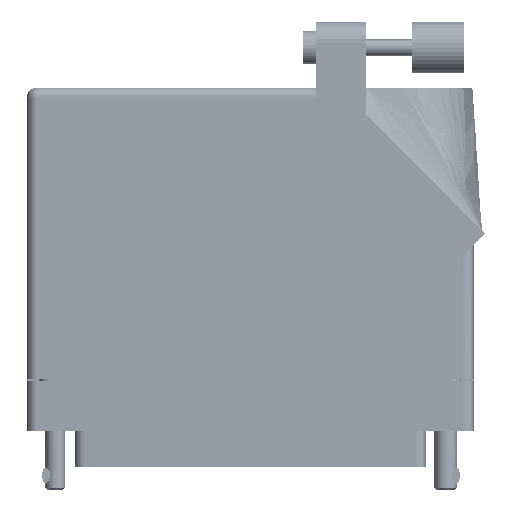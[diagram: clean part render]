
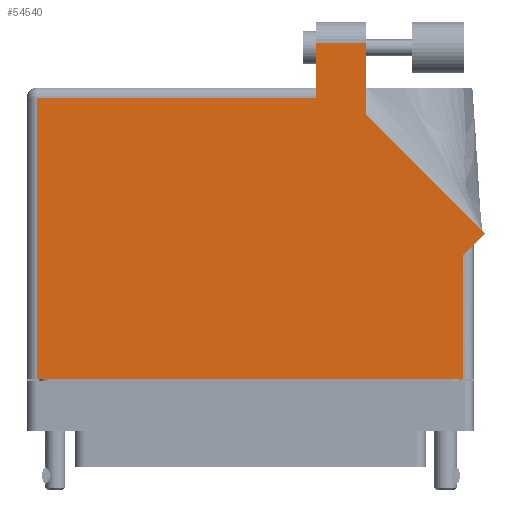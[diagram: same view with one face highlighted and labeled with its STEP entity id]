
A CAD part, front view. The second image highlights one B-rep face of the part: STEP entity #54540.
In plain terms, the highlighted face is planar.
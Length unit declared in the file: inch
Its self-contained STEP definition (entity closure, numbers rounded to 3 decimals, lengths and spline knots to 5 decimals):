
#1193 = CARTESIAN_POINT ( 'NONE',  ( -1.297, -0.1, 0.617 ) ) ;
#1477 = DIRECTION ( 'NONE',  ( -0.707, 0.707, 0. ) ) ;
#1693 = DIRECTION ( 'NONE',  ( -1., 0., 0. ) ) ;
#4612 = CARTESIAN_POINT ( 'NONE',  ( 1.297, 0.653, 0.617 ) ) ;
#4643 = VERTEX_POINT ( 'NONE', #49064 ) ;
#9513 = EDGE_CURVE ( 'NONE', #53875, #79108, #11971, .T. ) ;
#10270 = ORIENTED_EDGE ( 'NONE', *, *, #74179, .T. ) ;
#11971 = LINE ( 'NONE', #51084, #12599 ) ;
#12599 = VECTOR ( 'NONE', #78226, 39.37008 ) ;
#13262 = DIRECTION ( 'NONE',  ( 0., -1., 0. ) ) ;
#16221 = CARTESIAN_POINT ( 'NONE',  ( 0.706, 1.50942, 0.617 ) ) ;
#16449 = CARTESIAN_POINT ( 'NONE',  ( 1.297, -0.1, 0.617 ) ) ;
#17113 = EDGE_CURVE ( 'NONE', #79108, #62182, #32589, .T. ) ;
#20006 = PLANE ( 'NONE',  #80832 ) ;
#21875 = CARTESIAN_POINT ( 'NONE',  ( 1.297, 0.715, 0.617 ) ) ;
#22116 = CARTESIAN_POINT ( 'NONE',  ( -1.359, 1.613, 0.617 ) ) ;
#22216 = VECTOR ( 'NONE', #13262, 39.37008 ) ;
#22302 = EDGE_CURVE ( 'NONE', #73779, #49938, #82548, .T. ) ;
#24360 = DIRECTION ( 'NONE',  ( 0., -1., 0. ) ) ;
#24768 = CARTESIAN_POINT ( 'NONE',  ( 0.399, 1.675, 0.617 ) ) ;
#27907 = ORIENTED_EDGE ( 'NONE', *, *, #46086, .T. ) ;
#28222 = LINE ( 'NONE', #47340, #70638 ) ;
#28512 = LINE ( 'NONE', #22116, #83997 ) ;
#30144 = CARTESIAN_POINT ( 'NONE',  ( 0.706, 1.95, 0.617 ) ) ;
#32589 = LINE ( 'NONE', #78020, #60266 ) ;
#33393 = LINE ( 'NONE', #21875, #48167 ) ;
#34362 = ORIENTED_EDGE ( 'NONE', *, *, #9513, .T. ) ;
#41122 = VECTOR ( 'NONE', #69259, 39.37008 ) ;
#44297 = EDGE_LOOP ( 'NONE', ( #10270, #51695, #61561, #45291, #63371, #27907, #79459, #34362, #70894 ) ) ;
#44699 = EDGE_CURVE ( 'NONE', #55662, #73779, #28512, .T. ) ;
#45048 = VECTOR ( 'NONE', #78304, 39.37008 ) ;
#45291 = ORIENTED_EDGE ( 'NONE', *, *, #44699, .T. ) ;
#45940 = DIRECTION ( 'NONE',  ( 0., 0., -1. ) ) ;
#46086 = EDGE_CURVE ( 'NONE', #49938, #59798, #28222, .T. ) ;
#47340 = CARTESIAN_POINT ( 'NONE',  ( -1.359, -0.1, 0.617 ) ) ;
#47799 = DIRECTION ( 'NONE',  ( 0., 1., 0. ) ) ;
#48047 = DIRECTION ( 'NONE',  ( -1., 0., 0. ) ) ;
#48167 = VECTOR ( 'NONE', #47799, 39.37008 ) ;
#49064 = CARTESIAN_POINT ( 'NONE',  ( 0.399, 1.95, 0.617 ) ) ;
#49938 = VERTEX_POINT ( 'NONE', #1193 ) ;
#51084 = CARTESIAN_POINT ( 'NONE',  ( 1.359, 0.715, 0.617 ) ) ;
#51695 = ORIENTED_EDGE ( 'NONE', *, *, #59368, .T. ) ;
#52888 = DIRECTION ( 'NONE',  ( 1., 0., 0. ) ) ;
#52940 = CARTESIAN_POINT ( 'NONE',  ( 1.42971, 0.78571, 0.617 ) ) ;
#53875 = VERTEX_POINT ( 'NONE', #4612 ) ;
#54540 = ADVANCED_FACE ( 'NONE', ( #72256 ), #20006, .F. ) ;
#55662 = VERTEX_POINT ( 'NONE', #81338 ) ;
#57773 = CARTESIAN_POINT ( 'NONE',  ( 0.399, 1.95, 0.617 ) ) ;
#58762 = CARTESIAN_POINT ( 'NONE',  ( 0.706, 1.50942, 0.617 ) ) ;
#59368 = EDGE_CURVE ( 'NONE', #66008, #4643, #75627, .T. ) ;
#59798 = VERTEX_POINT ( 'NONE', #16449 ) ;
#60266 = VECTOR ( 'NONE', #1477, 39.37008 ) ;
#60312 = VECTOR ( 'NONE', #24360, 39.37008 ) ;
#61561 = ORIENTED_EDGE ( 'NONE', *, *, #83918, .T. ) ;
#62182 = VERTEX_POINT ( 'NONE', #16221 ) ;
#63371 = ORIENTED_EDGE ( 'NONE', *, *, #22302, .T. ) ;
#66008 = VERTEX_POINT ( 'NONE', #30144 ) ;
#69259 = DIRECTION ( 'NONE',  ( -1., 0., 0. ) ) ;
#70638 = VECTOR ( 'NONE', #52888, 39.37008 ) ;
#70894 = ORIENTED_EDGE ( 'NONE', *, *, #17113, .T. ) ;
#72256 = FACE_OUTER_BOUND ( 'NONE', #44297, .T. ) ;
#72444 = CARTESIAN_POINT ( 'NONE',  ( -1.297, 1.613, 0.617 ) ) ;
#72692 = CARTESIAN_POINT ( 'NONE',  ( -1.359, 1.675, 0.617 ) ) ;
#73779 = VERTEX_POINT ( 'NONE', #72444 ) ;
#73939 = LINE ( 'NONE', #58762, #45048 ) ;
#74179 = EDGE_CURVE ( 'NONE', #62182, #66008, #73939, .T. ) ;
#75627 = LINE ( 'NONE', #57773, #41122 ) ;
#78020 = CARTESIAN_POINT ( 'NONE',  ( 1.42971, 0.78571, 0.617 ) ) ;
#78226 = DIRECTION ( 'NONE',  ( 0.707, 0.707, 0. ) ) ;
#78304 = DIRECTION ( 'NONE',  ( 0., 1., 0. ) ) ;
#79081 = EDGE_CURVE ( 'NONE', #59798, #53875, #33393, .T. ) ;
#79108 = VERTEX_POINT ( 'NONE', #52940 ) ;
#79459 = ORIENTED_EDGE ( 'NONE', *, *, #79081, .T. ) ;
#80832 = AXIS2_PLACEMENT_3D ( 'NONE', #72692, #45940, #1693 ) ;
#81338 = CARTESIAN_POINT ( 'NONE',  ( 0.399, 1.613, 0.617 ) ) ;
#81694 = CARTESIAN_POINT ( 'NONE',  ( -1.297, -0.1, 0.617 ) ) ;
#82548 = LINE ( 'NONE', #81694, #60312 ) ;
#83404 = LINE ( 'NONE', #24768, #22216 ) ;
#83918 = EDGE_CURVE ( 'NONE', #4643, #55662, #83404, .T. ) ;
#83997 = VECTOR ( 'NONE', #48047, 39.37008 ) ;
